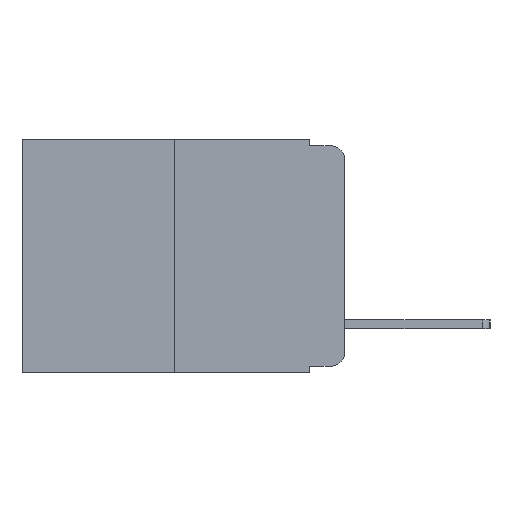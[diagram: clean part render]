
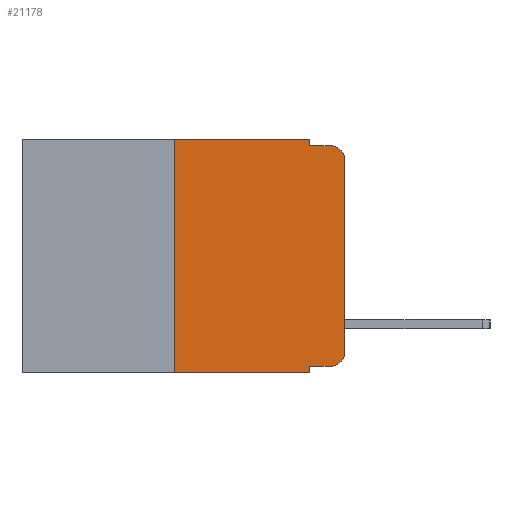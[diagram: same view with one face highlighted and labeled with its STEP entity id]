
A CAD part, left-side view. The second image highlights one B-rep face of the part: STEP entity #21178.
In plain terms, the highlighted planar face has unit normal (-1, 0, 0).
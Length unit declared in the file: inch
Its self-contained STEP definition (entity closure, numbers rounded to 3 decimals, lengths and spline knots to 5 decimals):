
#1252 = CARTESIAN_POINT ( 'NONE',  ( 0., 0.051, -0.01 ) ) ;
#1289 = ORIENTED_EDGE ( 'NONE', *, *, #19810, .F. ) ;
#1306 = EDGE_CURVE ( 'NONE', #4169, #13861, #3940, .T. ) ;
#1899 = DIRECTION ( 'NONE',  ( 0., -1., 0. ) ) ;
#2031 = EDGE_CURVE ( 'NONE', #13924, #13850, #20801, .T. ) ;
#2264 = LINE ( 'NONE', #10844, #19441 ) ;
#2266 = VECTOR ( 'NONE', #13724, 39.37008 ) ;
#2804 = LINE ( 'NONE', #11927, #2266 ) ;
#3572 = CARTESIAN_POINT ( 'NONE',  ( 0., 0.051, -0.01 ) ) ;
#3582 = EDGE_CURVE ( 'NONE', #14946, #13850, #2804, .T. ) ;
#3814 = LINE ( 'NONE', #3572, #4369 ) ;
#3940 = CIRCLE ( 'NONE', #20411, 0.02 ) ;
#4011 = DIRECTION ( 'NONE',  ( -1., 0., 0. ) ) ;
#4114 = DIRECTION ( 'NONE',  ( 1., 0., 0. ) ) ;
#4169 = VERTEX_POINT ( 'NONE', #9905 ) ;
#4369 = VECTOR ( 'NONE', #1899, 39.37008 ) ;
#4828 = EDGE_CURVE ( 'NONE', #13591, #16443, #17640, .T. ) ;
#5219 = LINE ( 'NONE', #10594, #13492 ) ;
#5324 = ORIENTED_EDGE ( 'NONE', *, *, #8681, .T. ) ;
#5510 = ORIENTED_EDGE ( 'NONE', *, *, #2031, .F. ) ;
#5595 = DIRECTION ( 'NONE',  ( 0., -1., 0. ) ) ;
#6035 = LINE ( 'NONE', #16137, #14332 ) ;
#6623 = FACE_OUTER_BOUND ( 'NONE', #17448, .T. ) ;
#6651 = CARTESIAN_POINT ( 'NONE',  ( 0., 0.051, -0.333 ) ) ;
#6988 = ORIENTED_EDGE ( 'NONE', *, *, #1306, .T. ) ;
#7619 = CARTESIAN_POINT ( 'NONE',  ( 0., 0.25, -0.343 ) ) ;
#7774 = AXIS2_PLACEMENT_3D ( 'NONE', #14033, #4114, #15738 ) ;
#7930 = DIRECTION ( 'NONE',  ( 0., 0., 1. ) ) ;
#8655 = CARTESIAN_POINT ( 'NONE',  ( 0., 0., -0.313 ) ) ;
#8681 = EDGE_CURVE ( 'NONE', #16443, #4169, #6035, .T. ) ;
#8821 = DIRECTION ( 'NONE',  ( 0., 0., -1. ) ) ;
#9000 = DIRECTION ( 'NONE',  ( 0., 0., -1. ) ) ;
#9034 = PLANE ( 'NONE',  #7774 ) ;
#9254 = DIRECTION ( 'NONE',  ( 0., -1., 0. ) ) ;
#9374 = CARTESIAN_POINT ( 'NONE',  ( 0., 0.02, -0.313 ) ) ;
#9662 = CARTESIAN_POINT ( 'NONE',  ( 0., 0.051, 0. ) ) ;
#9707 = DIRECTION ( 'NONE',  ( 0., 0., -1. ) ) ;
#9824 = LINE ( 'NONE', #17110, #18178 ) ;
#9905 = CARTESIAN_POINT ( 'NONE',  ( 0., 0., -0.03 ) ) ;
#10594 = CARTESIAN_POINT ( 'NONE',  ( 0., 0.473, 0. ) ) ;
#10844 = CARTESIAN_POINT ( 'NONE',  ( 0., 0.051, -0.333 ) ) ;
#11290 = ORIENTED_EDGE ( 'NONE', *, *, #4828, .T. ) ;
#11927 = CARTESIAN_POINT ( 'NONE',  ( 0., 0.473, -0.343 ) ) ;
#12065 = AXIS2_PLACEMENT_3D ( 'NONE', #9374, #4011, #19994 ) ;
#12090 = CARTESIAN_POINT ( 'NONE',  ( 0., 0.25, 0. ) ) ;
#12237 = ORIENTED_EDGE ( 'NONE', *, *, #19450, .T. ) ;
#13094 = VECTOR ( 'NONE', #8821, 39.37008 ) ;
#13492 = VECTOR ( 'NONE', #5595, 39.37008 ) ;
#13554 = ORIENTED_EDGE ( 'NONE', *, *, #3582, .T. ) ;
#13591 = VERTEX_POINT ( 'NONE', #15742 ) ;
#13724 = DIRECTION ( 'NONE',  ( 0., -1., 0. ) ) ;
#13729 = CARTESIAN_POINT ( 'NONE',  ( 0., 0.051, 0. ) ) ;
#13850 = VERTEX_POINT ( 'NONE', #14778 ) ;
#13861 = VERTEX_POINT ( 'NONE', #18158 ) ;
#13924 = VERTEX_POINT ( 'NONE', #6651 ) ;
#14033 = CARTESIAN_POINT ( 'NONE',  ( 0., 0.473, 0. ) ) ;
#14089 = DIRECTION ( 'NONE',  ( -1., 0., 0. ) ) ;
#14332 = VECTOR ( 'NONE', #7930, 39.37008 ) ;
#14383 = VERTEX_POINT ( 'NONE', #1252 ) ;
#14778 = CARTESIAN_POINT ( 'NONE',  ( 0., 0.051, -0.343 ) ) ;
#14782 = EDGE_CURVE ( 'NONE', #18399, #15209, #5219, .T. ) ;
#14946 = VERTEX_POINT ( 'NONE', #7619 ) ;
#15209 = VERTEX_POINT ( 'NONE', #18600 ) ;
#15738 = DIRECTION ( 'NONE',  ( 0., 0., -1. ) ) ;
#15742 = CARTESIAN_POINT ( 'NONE',  ( 0., 0.02, -0.333 ) ) ;
#15880 = VECTOR ( 'NONE', #9707, 39.37008 ) ;
#16137 = CARTESIAN_POINT ( 'NONE',  ( 0., 0., 0. ) ) ;
#16443 = VERTEX_POINT ( 'NONE', #8655 ) ;
#16523 = ORIENTED_EDGE ( 'NONE', *, *, #14782, .F. ) ;
#16547 = ORIENTED_EDGE ( 'NONE', *, *, #21084, .F. ) ;
#17098 = CARTESIAN_POINT ( 'NONE',  ( 0., 0.02, -0.03 ) ) ;
#17110 = CARTESIAN_POINT ( 'NONE',  ( 0., 0.25, 0. ) ) ;
#17448 = EDGE_LOOP ( 'NONE', ( #5324, #6988, #1289, #16547, #16523, #19687, #13554, #5510, #12237, #11290 ) ) ;
#17561 = LINE ( 'NONE', #13729, #13094 ) ;
#17640 = CIRCLE ( 'NONE', #12065, 0.02 ) ;
#18158 = CARTESIAN_POINT ( 'NONE',  ( 0., 0.02, -0.01 ) ) ;
#18178 = VECTOR ( 'NONE', #18784, 39.37008 ) ;
#18399 = VERTEX_POINT ( 'NONE', #12090 ) ;
#18600 = CARTESIAN_POINT ( 'NONE',  ( 0., 0.051, 0. ) ) ;
#18784 = DIRECTION ( 'NONE',  ( 0., 0., 1. ) ) ;
#19288 = EDGE_CURVE ( 'NONE', #14946, #18399, #9824, .T. ) ;
#19441 = VECTOR ( 'NONE', #9254, 39.37008 ) ;
#19450 = EDGE_CURVE ( 'NONE', #13924, #13591, #2264, .T. ) ;
#19687 = ORIENTED_EDGE ( 'NONE', *, *, #19288, .F. ) ;
#19810 = EDGE_CURVE ( 'NONE', #14383, #13861, #3814, .T. ) ;
#19994 = DIRECTION ( 'NONE',  ( 0., 0., -1. ) ) ;
#20411 = AXIS2_PLACEMENT_3D ( 'NONE', #17098, #14089, #9000 ) ;
#20801 = LINE ( 'NONE', #9662, #15880 ) ;
#21084 = EDGE_CURVE ( 'NONE', #15209, #14383, #17561, .T. ) ;
#21178 = ADVANCED_FACE ( 'NONE', ( #6623 ), #9034, .F. ) ;
